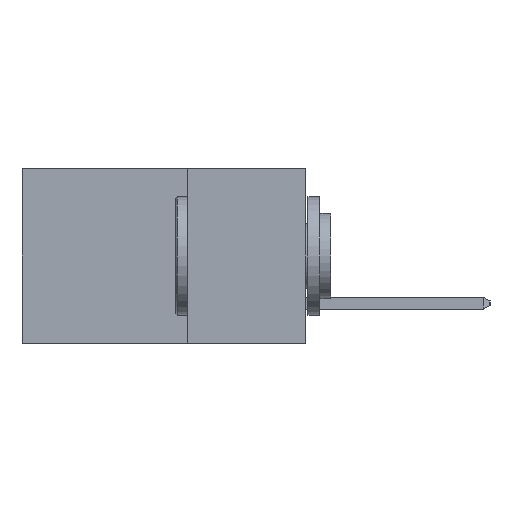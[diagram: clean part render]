
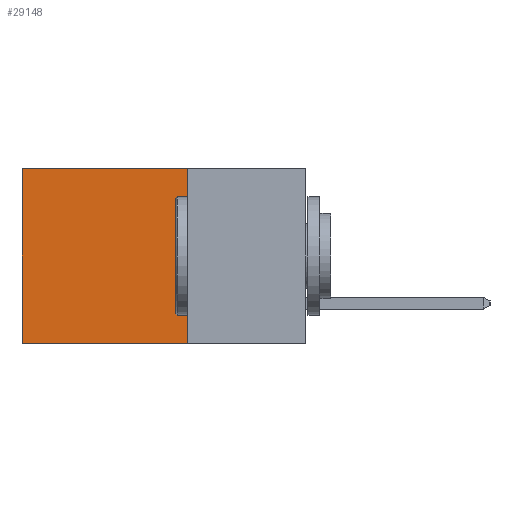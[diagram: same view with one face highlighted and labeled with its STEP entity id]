
A CAD part, left-side view. The second image highlights one B-rep face of the part: STEP entity #29148.
In plain terms, the highlighted planar face has unit normal (-1, 0, 0).
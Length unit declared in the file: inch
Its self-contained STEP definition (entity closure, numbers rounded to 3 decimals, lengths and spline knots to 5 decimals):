
#935 = DIRECTION ( 'NONE',  ( 0., 0., -1. ) ) ;
#938 = CARTESIAN_POINT ( 'NONE',  ( 0.298, 0.6, 0. ) ) ;
#1155 = VECTOR ( 'NONE', #20228, 39.37008 ) ;
#1810 = EDGE_CURVE ( 'NONE', #7636, #12356, #32156, .T. ) ;
#3535 = DIRECTION ( 'NONE',  ( 0., 0., -1. ) ) ;
#3843 = CARTESIAN_POINT ( 'NONE',  ( 0.298, 0.6, 0. ) ) ;
#7498 = VERTEX_POINT ( 'NONE', #17954 ) ;
#7636 = VERTEX_POINT ( 'NONE', #13429 ) ;
#8455 = ORIENTED_EDGE ( 'NONE', *, *, #1810, .F. ) ;
#9443 = LINE ( 'NONE', #24794, #29349 ) ;
#10513 = ORIENTED_EDGE ( 'NONE', *, *, #19354, .F. ) ;
#10706 = ORIENTED_EDGE ( 'NONE', *, *, #19724, .T. ) ;
#11370 = AXIS2_PLACEMENT_3D ( 'NONE', #32104, #14939, #32205 ) ;
#11724 = VERTEX_POINT ( 'NONE', #3843 ) ;
#12264 = DIRECTION ( 'NONE',  ( 0., 1., 0. ) ) ;
#12356 = VERTEX_POINT ( 'NONE', #16611 ) ;
#12368 = PLANE ( 'NONE',  #11370 ) ;
#13429 = CARTESIAN_POINT ( 'NONE',  ( 0.298, 0.25, 0. ) ) ;
#13958 = VECTOR ( 'NONE', #935, 39.37008 ) ;
#14939 = DIRECTION ( 'NONE',  ( 1., 0., 0. ) ) ;
#16611 = CARTESIAN_POINT ( 'NONE',  ( 0.298, 0.25, -0.37 ) ) ;
#16929 = LINE ( 'NONE', #938, #29320 ) ;
#17281 = EDGE_CURVE ( 'NONE', #7636, #11724, #28002, .T. ) ;
#17489 = EDGE_LOOP ( 'NONE', ( #10706, #10513, #8455, #24006 ) ) ;
#17954 = CARTESIAN_POINT ( 'NONE',  ( 0.298, 0.6, -0.37 ) ) ;
#19354 = EDGE_CURVE ( 'NONE', #12356, #7498, #9443, .T. ) ;
#19724 = EDGE_CURVE ( 'NONE', #11724, #7498, #16929, .T. ) ;
#20228 = DIRECTION ( 'NONE',  ( 0., 1., 0. ) ) ;
#23755 = CARTESIAN_POINT ( 'NONE',  ( 0.298, 0.25, 0. ) ) ;
#24006 = ORIENTED_EDGE ( 'NONE', *, *, #17281, .T. ) ;
#24794 = CARTESIAN_POINT ( 'NONE',  ( 0.298, 0.25, -0.37 ) ) ;
#28002 = LINE ( 'NONE', #32453, #1155 ) ;
#29148 = ADVANCED_FACE ( 'NONE', ( #31742 ), #12368, .F. ) ;
#29320 = VECTOR ( 'NONE', #3535, 39.37008 ) ;
#29349 = VECTOR ( 'NONE', #12264, 39.37008 ) ;
#31742 = FACE_OUTER_BOUND ( 'NONE', #17489, .T. ) ;
#32104 = CARTESIAN_POINT ( 'NONE',  ( 0.298, 0.25, 0. ) ) ;
#32156 = LINE ( 'NONE', #23755, #13958 ) ;
#32205 = DIRECTION ( 'NONE',  ( 0., 0., -1. ) ) ;
#32453 = CARTESIAN_POINT ( 'NONE',  ( 0.298, 0.25, 0. ) ) ;
